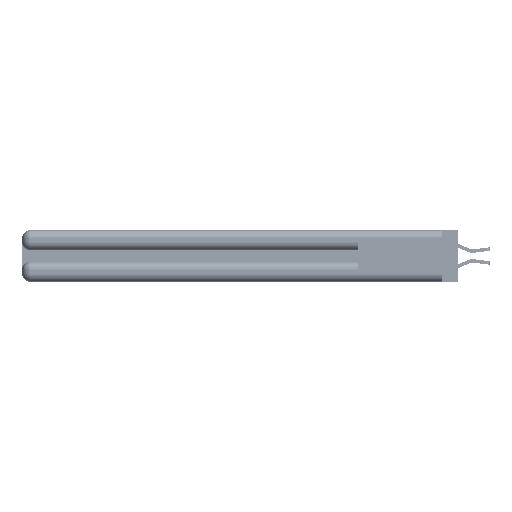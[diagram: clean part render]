
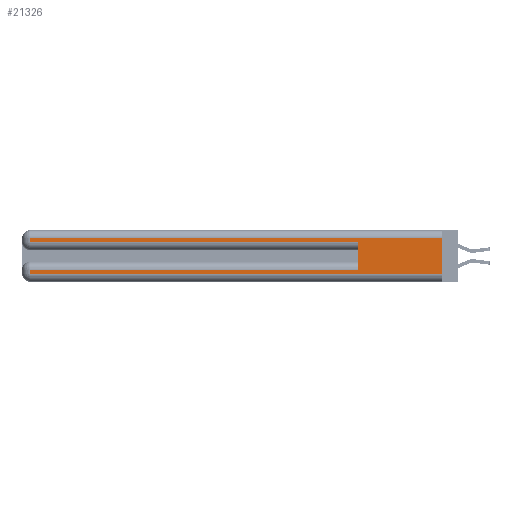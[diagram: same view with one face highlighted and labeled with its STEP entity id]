
A CAD part, left-side view. The second image highlights one B-rep face of the part: STEP entity #21326.
In plain terms, the highlighted planar face has unit normal (-1, 0, 0).
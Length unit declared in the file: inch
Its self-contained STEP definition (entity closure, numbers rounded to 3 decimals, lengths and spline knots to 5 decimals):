
#2 = VERTEX_POINT ( 'NONE', #19033 ) ;
#340 = VERTEX_POINT ( 'NONE', #7699 ) ;
#433 = DIRECTION ( 'NONE',  ( 0., 0., -1. ) ) ;
#680 = CARTESIAN_POINT ( 'NONE',  ( 0., 0., 0.06 ) ) ;
#1329 = ORIENTED_EDGE ( 'NONE', *, *, #1634, .T. ) ;
#1634 = EDGE_CURVE ( 'NONE', #27473, #340, #39158, .T. ) ;
#2641 = LINE ( 'NONE', #680, #19097 ) ;
#4042 = DIRECTION ( 'NONE',  ( 0., -1., 0. ) ) ;
#4313 = ORIENTED_EDGE ( 'NONE', *, *, #16540, .F. ) ;
#4326 = VECTOR ( 'NONE', #22891, 39.37008 ) ;
#4939 = VECTOR ( 'NONE', #21936, 39.37008 ) ;
#5554 = CARTESIAN_POINT ( 'NONE',  ( 0., 2.94, 0.37 ) ) ;
#6889 = DIRECTION ( 'NONE',  ( 0., 1., 0. ) ) ;
#6979 = AXIS2_PLACEMENT_3D ( 'NONE', #39813, #20203, #433 ) ;
#7628 = DIRECTION ( 'NONE',  ( 0., 0., -1. ) ) ;
#7699 = CARTESIAN_POINT ( 'NONE',  ( 0., 2.94, 0.06 ) ) ;
#10178 = VECTOR ( 'NONE', #6889, 39.37008 ) ;
#10261 = PLANE ( 'NONE',  #6979 ) ;
#11402 = LINE ( 'NONE', #22802, #35556 ) ;
#12136 = FACE_OUTER_BOUND ( 'NONE', #16194, .T. ) ;
#13004 = VECTOR ( 'NONE', #7628, 39.37008 ) ;
#13863 = CARTESIAN_POINT ( 'NONE',  ( 0., 0.6, 0.285 ) ) ;
#15259 = CARTESIAN_POINT ( 'NONE',  ( 0., 0.6, 0.085 ) ) ;
#16194 = EDGE_LOOP ( 'NONE', ( #4313, #42258, #32043, #40212, #42325, #37704, #1329, #32632 ) ) ;
#16477 = VECTOR ( 'NONE', #41437, 39.37008 ) ;
#16540 = EDGE_CURVE ( 'NONE', #34272, #2, #11402, .T. ) ;
#18544 = EDGE_CURVE ( 'NONE', #33955, #27473, #18919, .T. ) ;
#18919 = LINE ( 'NONE', #39563, #10178 ) ;
#19033 = CARTESIAN_POINT ( 'NONE',  ( 0., 0., 0.06 ) ) ;
#19097 = VECTOR ( 'NONE', #4042, 39.37008 ) ;
#20203 = DIRECTION ( 'NONE',  ( 1., 0., 0. ) ) ;
#20519 = LINE ( 'NONE', #25886, #28209 ) ;
#21326 = ADVANCED_FACE ( 'NONE', ( #12136 ), #10261, .F. ) ;
#21936 = DIRECTION ( 'NONE',  ( 0., 0., -1. ) ) ;
#22423 = EDGE_CURVE ( 'NONE', #34272, #34941, #23869, .T. ) ;
#22496 = VERTEX_POINT ( 'NONE', #26782 ) ;
#22709 = DIRECTION ( 'NONE',  ( 0., -1., 0. ) ) ;
#22802 = CARTESIAN_POINT ( 'NONE',  ( 0., 0., 0.37 ) ) ;
#22891 = DIRECTION ( 'NONE',  ( 0., 1., 0. ) ) ;
#23869 = LINE ( 'NONE', #35962, #4326 ) ;
#25190 = LINE ( 'NONE', #38154, #16477 ) ;
#25886 = CARTESIAN_POINT ( 'NONE',  ( 0., 0., 0.285 ) ) ;
#26026 = EDGE_CURVE ( 'NONE', #33955, #27062, #25190, .T. ) ;
#26782 = CARTESIAN_POINT ( 'NONE',  ( 0., 2.94, 0.285 ) ) ;
#27062 = VERTEX_POINT ( 'NONE', #13863 ) ;
#27273 = CARTESIAN_POINT ( 'NONE',  ( 0., 2.94, 0.37 ) ) ;
#27473 = VERTEX_POINT ( 'NONE', #38616 ) ;
#27554 = EDGE_CURVE ( 'NONE', #22496, #27062, #20519, .T. ) ;
#28209 = VECTOR ( 'NONE', #22709, 39.37008 ) ;
#30452 = CARTESIAN_POINT ( 'NONE',  ( 0., 0., 0.31 ) ) ;
#31741 = EDGE_CURVE ( 'NONE', #340, #2, #2641, .T. ) ;
#32043 = ORIENTED_EDGE ( 'NONE', *, *, #34497, .T. ) ;
#32632 = ORIENTED_EDGE ( 'NONE', *, *, #31741, .T. ) ;
#33955 = VERTEX_POINT ( 'NONE', #15259 ) ;
#34113 = CARTESIAN_POINT ( 'NONE',  ( 0., 2.94, 0.31 ) ) ;
#34272 = VERTEX_POINT ( 'NONE', #30452 ) ;
#34497 = EDGE_CURVE ( 'NONE', #34941, #22496, #38818, .T. ) ;
#34941 = VERTEX_POINT ( 'NONE', #34113 ) ;
#35556 = VECTOR ( 'NONE', #42377, 39.37008 ) ;
#35962 = CARTESIAN_POINT ( 'NONE',  ( 0., 0., 0.31 ) ) ;
#37704 = ORIENTED_EDGE ( 'NONE', *, *, #18544, .T. ) ;
#38154 = CARTESIAN_POINT ( 'NONE',  ( 0., 0.6, 0.145 ) ) ;
#38616 = CARTESIAN_POINT ( 'NONE',  ( 0., 2.94, 0.085 ) ) ;
#38818 = LINE ( 'NONE', #5554, #4939 ) ;
#39158 = LINE ( 'NONE', #27273, #13004 ) ;
#39563 = CARTESIAN_POINT ( 'NONE',  ( 0., 0., 0.085 ) ) ;
#39813 = CARTESIAN_POINT ( 'NONE',  ( 0., 0., 0.37 ) ) ;
#40212 = ORIENTED_EDGE ( 'NONE', *, *, #27554, .T. ) ;
#41437 = DIRECTION ( 'NONE',  ( 0., 0., 1. ) ) ;
#42258 = ORIENTED_EDGE ( 'NONE', *, *, #22423, .T. ) ;
#42325 = ORIENTED_EDGE ( 'NONE', *, *, #26026, .F. ) ;
#42377 = DIRECTION ( 'NONE',  ( 0., 0., -1. ) ) ;
